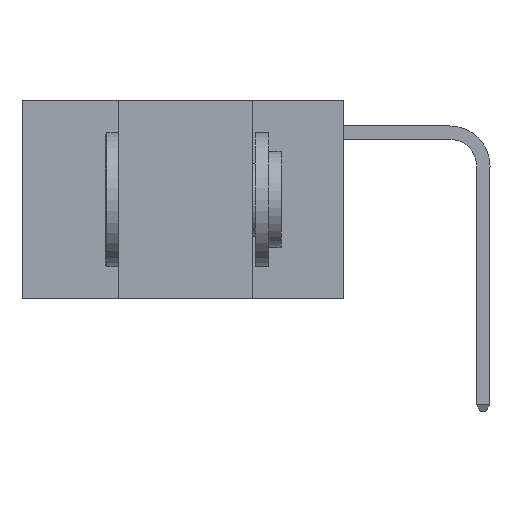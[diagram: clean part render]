
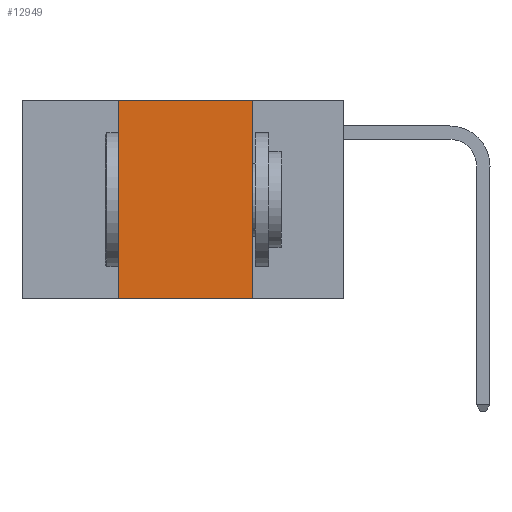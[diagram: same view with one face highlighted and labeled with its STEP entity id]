
A CAD part, left-side view. The second image highlights one B-rep face of the part: STEP entity #12949.
In plain terms, the highlighted planar face has unit normal (-1, 0, 0).
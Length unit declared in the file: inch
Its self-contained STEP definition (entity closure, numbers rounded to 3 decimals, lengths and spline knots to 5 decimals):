
#184 = EDGE_CURVE ( 'NONE', #10498, #1625, #597, .T. ) ;
#546 = VECTOR ( 'NONE', #7803, 39.37008 ) ;
#597 = LINE ( 'NONE', #8548, #546 ) ;
#982 = DIRECTION ( 'NONE',  ( 0., 0., 1. ) ) ;
#996 = VECTOR ( 'NONE', #982, 39.37008 ) ;
#1625 = VERTEX_POINT ( 'NONE', #14422 ) ;
#2138 = DIRECTION ( 'NONE',  ( 0., 0., -1. ) ) ;
#2176 = LINE ( 'NONE', #4622, #13917 ) ;
#2981 = CARTESIAN_POINT ( 'NONE',  ( 0., 0.6, 0. ) ) ;
#3116 = VECTOR ( 'NONE', #2138, 39.37008 ) ;
#3407 = CARTESIAN_POINT ( 'NONE',  ( 0., 0.17, 0. ) ) ;
#3540 = LINE ( 'NONE', #3407, #3116 ) ;
#4297 = DIRECTION ( 'NONE',  ( 0., 0., -1. ) ) ;
#4622 = CARTESIAN_POINT ( 'NONE',  ( 0., 0.6, 0. ) ) ;
#6173 = EDGE_CURVE ( 'NONE', #7794, #1625, #3540, .T. ) ;
#6256 = EDGE_CURVE ( 'NONE', #10498, #8990, #14000, .T. ) ;
#6431 = CARTESIAN_POINT ( 'NONE',  ( 0., 0.17, 0. ) ) ;
#7794 = VERTEX_POINT ( 'NONE', #6431 ) ;
#7803 = DIRECTION ( 'NONE',  ( 0., -1., 0. ) ) ;
#8548 = CARTESIAN_POINT ( 'NONE',  ( 0., 0.6, -0.37 ) ) ;
#8566 = CARTESIAN_POINT ( 'NONE',  ( 0., 0.42, -0.37 ) ) ;
#8990 = VERTEX_POINT ( 'NONE', #12509 ) ;
#9232 = PLANE ( 'NONE',  #14696 ) ;
#10498 = VERTEX_POINT ( 'NONE', #8566 ) ;
#10603 = FACE_OUTER_BOUND ( 'NONE', #10697, .T. ) ;
#10697 = EDGE_LOOP ( 'NONE', ( #10970, #11116, #11229, #11567 ) ) ;
#10970 = ORIENTED_EDGE ( 'NONE', *, *, #6173, .F. ) ;
#11116 = ORIENTED_EDGE ( 'NONE', *, *, #12167, .F. ) ;
#11229 = ORIENTED_EDGE ( 'NONE', *, *, #6256, .F. ) ;
#11567 = ORIENTED_EDGE ( 'NONE', *, *, #184, .T. ) ;
#11646 = DIRECTION ( 'NONE',  ( 1., 0., 0. ) ) ;
#11906 = DIRECTION ( 'NONE',  ( 0., -1., 0. ) ) ;
#12167 = EDGE_CURVE ( 'NONE', #8990, #7794, #2176, .T. ) ;
#12509 = CARTESIAN_POINT ( 'NONE',  ( 0., 0.42, 0. ) ) ;
#12949 = ADVANCED_FACE ( 'NONE', ( #10603 ), #9232, .F. ) ;
#13917 = VECTOR ( 'NONE', #11906, 39.37008 ) ;
#14000 = LINE ( 'NONE', #15363, #996 ) ;
#14422 = CARTESIAN_POINT ( 'NONE',  ( 0., 0.17, -0.37 ) ) ;
#14696 = AXIS2_PLACEMENT_3D ( 'NONE', #2981, #11646, #4297 ) ;
#15363 = CARTESIAN_POINT ( 'NONE',  ( 0., 0.42, 0. ) ) ;
